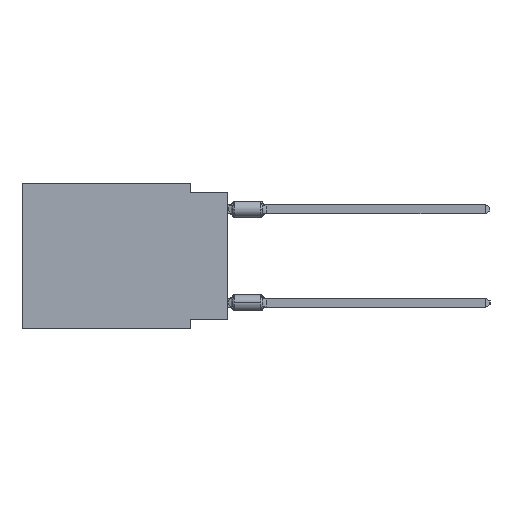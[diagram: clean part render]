
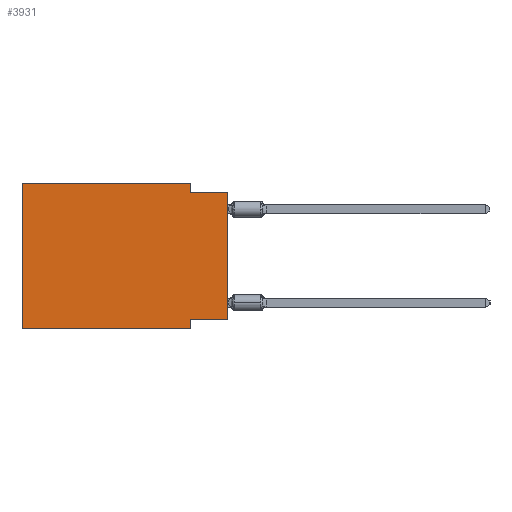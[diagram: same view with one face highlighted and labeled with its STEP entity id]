
A CAD part, left-side view. The second image highlights one B-rep face of the part: STEP entity #3931.
In plain terms, the highlighted planar face has unit normal (-1, 0, 0).
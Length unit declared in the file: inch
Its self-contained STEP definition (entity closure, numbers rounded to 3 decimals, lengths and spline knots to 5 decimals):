
#539 = EDGE_LOOP ( 'NONE', ( #19270, #21577, #29902, #28393, #18372, #21566, #25333, #3554 ) ) ;
#1220 = CARTESIAN_POINT ( 'NONE',  ( 0., 0.55, 0. ) ) ;
#1824 = CARTESIAN_POINT ( 'NONE',  ( 0., 0., 0. ) ) ;
#2499 = LINE ( 'NONE', #8059, #31676 ) ;
#3554 = ORIENTED_EDGE ( 'NONE', *, *, #27166, .F. ) ;
#3931 = ADVANCED_FACE ( 'NONE', ( #6433 ), #12338, .F. ) ;
#4083 = CARTESIAN_POINT ( 'NONE',  ( 0., 0.55, 0. ) ) ;
#4135 = CARTESIAN_POINT ( 'NONE',  ( 0., 0.1, -0.39 ) ) ;
#4173 = DIRECTION ( 'NONE',  ( 0., 0., 1. ) ) ;
#4488 = DIRECTION ( 'NONE',  ( 0., 0., -1. ) ) ;
#4910 = CARTESIAN_POINT ( 'NONE',  ( 0., 0.55, 0. ) ) ;
#5055 = VECTOR ( 'NONE', #31963, 39.37008 ) ;
#5592 = LINE ( 'NONE', #21868, #12802 ) ;
#6378 = CARTESIAN_POINT ( 'NONE',  ( 0., 0.1, -0.025 ) ) ;
#6433 = FACE_OUTER_BOUND ( 'NONE', #539, .T. ) ;
#6774 = LINE ( 'NONE', #17683, #6855 ) ;
#6855 = VECTOR ( 'NONE', #15013, 39.37008 ) ;
#6904 = DIRECTION ( 'NONE',  ( 0., -1., 0. ) ) ;
#6952 = CARTESIAN_POINT ( 'NONE',  ( 0., 0., -0.025 ) ) ;
#7223 = CARTESIAN_POINT ( 'NONE',  ( 0., 0.55, -0.39 ) ) ;
#8059 = CARTESIAN_POINT ( 'NONE',  ( 0., 0.1, 0. ) ) ;
#9172 = CARTESIAN_POINT ( 'NONE',  ( 0., 0., -0.365 ) ) ;
#9490 = DIRECTION ( 'NONE',  ( 0., 0., -1. ) ) ;
#9961 = LINE ( 'NONE', #31822, #33245 ) ;
#10571 = DIRECTION ( 'NONE',  ( 0., 0., -1. ) ) ;
#12338 = PLANE ( 'NONE',  #26358 ) ;
#12802 = VECTOR ( 'NONE', #35121, 39.37008 ) ;
#13057 = VERTEX_POINT ( 'NONE', #26131 ) ;
#15013 = DIRECTION ( 'NONE',  ( 0., 0., 1. ) ) ;
#15591 = EDGE_CURVE ( 'NONE', #21128, #32569, #6774, .T. ) ;
#17174 = EDGE_CURVE ( 'NONE', #22598, #26118, #9961, .T. ) ;
#17683 = CARTESIAN_POINT ( 'NONE',  ( 0., 0.55, 0. ) ) ;
#18372 = ORIENTED_EDGE ( 'NONE', *, *, #15591, .F. ) ;
#19270 = ORIENTED_EDGE ( 'NONE', *, *, #33073, .T. ) ;
#19355 = CARTESIAN_POINT ( 'NONE',  ( 0., 0.1, 0. ) ) ;
#20415 = LINE ( 'NONE', #4135, #32816 ) ;
#21052 = CARTESIAN_POINT ( 'NONE',  ( 0., 0., -0.365 ) ) ;
#21128 = VERTEX_POINT ( 'NONE', #7223 ) ;
#21227 = DIRECTION ( 'NONE',  ( 0., 1., 0. ) ) ;
#21351 = VERTEX_POINT ( 'NONE', #9172 ) ;
#21566 = ORIENTED_EDGE ( 'NONE', *, *, #31818, .T. ) ;
#21577 = ORIENTED_EDGE ( 'NONE', *, *, #17174, .F. ) ;
#21868 = CARTESIAN_POINT ( 'NONE',  ( 0., 0.55, -0.39 ) ) ;
#22598 = VERTEX_POINT ( 'NONE', #6378 ) ;
#24055 = LINE ( 'NONE', #4910, #5055 ) ;
#24283 = LINE ( 'NONE', #21052, #25548 ) ;
#25031 = CARTESIAN_POINT ( 'NONE',  ( 0., 0.1, -0.39 ) ) ;
#25333 = ORIENTED_EDGE ( 'NONE', *, *, #33500, .F. ) ;
#25548 = VECTOR ( 'NONE', #21227, 39.37008 ) ;
#26118 = VERTEX_POINT ( 'NONE', #6952 ) ;
#26131 = CARTESIAN_POINT ( 'NONE',  ( 0., 0.1, -0.365 ) ) ;
#26358 = AXIS2_PLACEMENT_3D ( 'NONE', #1220, #30985, #9490 ) ;
#26875 = VERTEX_POINT ( 'NONE', #25031 ) ;
#27166 = EDGE_CURVE ( 'NONE', #21351, #13057, #24283, .T. ) ;
#27503 = EDGE_CURVE ( 'NONE', #32569, #31961, #24055, .T. ) ;
#28393 = ORIENTED_EDGE ( 'NONE', *, *, #27503, .F. ) ;
#28714 = LINE ( 'NONE', #1824, #34012 ) ;
#29902 = ORIENTED_EDGE ( 'NONE', *, *, #33531, .F. ) ;
#30985 = DIRECTION ( 'NONE',  ( 1., 0., 0. ) ) ;
#31676 = VECTOR ( 'NONE', #10571, 39.37008 ) ;
#31818 = EDGE_CURVE ( 'NONE', #21128, #26875, #5592, .T. ) ;
#31822 = CARTESIAN_POINT ( 'NONE',  ( 0., 0., -0.025 ) ) ;
#31961 = VERTEX_POINT ( 'NONE', #19355 ) ;
#31963 = DIRECTION ( 'NONE',  ( 0., -1., 0. ) ) ;
#32569 = VERTEX_POINT ( 'NONE', #4083 ) ;
#32816 = VECTOR ( 'NONE', #4488, 39.37008 ) ;
#33073 = EDGE_CURVE ( 'NONE', #21351, #26118, #28714, .T. ) ;
#33245 = VECTOR ( 'NONE', #6904, 39.37008 ) ;
#33500 = EDGE_CURVE ( 'NONE', #13057, #26875, #20415, .T. ) ;
#33531 = EDGE_CURVE ( 'NONE', #31961, #22598, #2499, .T. ) ;
#34012 = VECTOR ( 'NONE', #4173, 39.37008 ) ;
#35121 = DIRECTION ( 'NONE',  ( 0., -1., 0. ) ) ;
